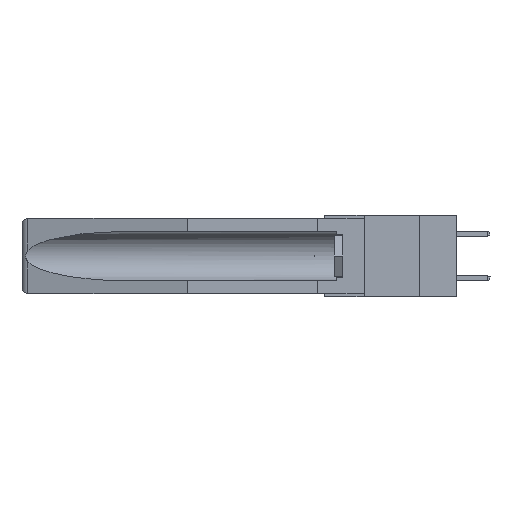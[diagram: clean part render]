
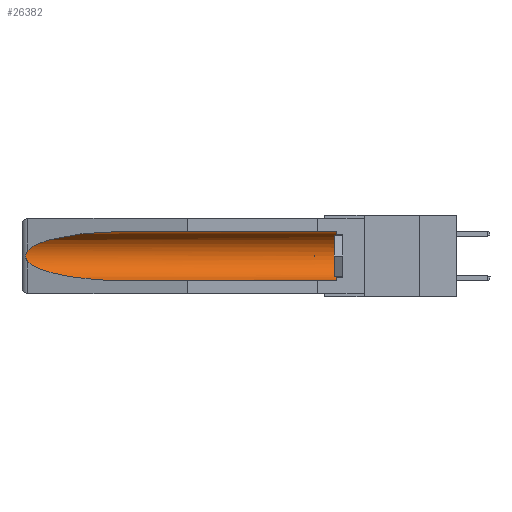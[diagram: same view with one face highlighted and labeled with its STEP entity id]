
A CAD part, left-side view. The second image highlights one B-rep face of the part: STEP entity #26382.
In plain terms, the highlighted cylindrical face has radius 2.857 mm (diameter 5.715 mm), a partial arc.
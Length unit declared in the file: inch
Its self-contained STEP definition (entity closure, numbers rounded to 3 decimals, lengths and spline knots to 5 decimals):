
#333 = DIRECTION ( 'NONE',  ( 0., 0., 1. ) ) ;
#480 = CARTESIAN_POINT ( 'NONE',  ( 0.155, 1.07973, -0.284 ) ) ;
#573 = EDGE_CURVE ( 'NONE', #24997, #14229, #4166, .T. ) ;
#666 = CARTESIAN_POINT ( 'NONE',  ( 0.26537, 1.52718, -0.14972 ) ) ;
#748 = VECTOR ( 'NONE', #4644, 39.37008 ) ;
#827 = LINE ( 'NONE', #33264, #28875 ) ;
#837 = ORIENTED_EDGE ( 'NONE', *, *, #14460, .T. ) ;
#1268 = CARTESIAN_POINT ( 'NONE',  ( 0.26537, 1.52718, -0.19328 ) ) ;
#1581 = CARTESIAN_POINT ( 'NONE',  ( 0.155, 0.126, -0.059 ) ) ;
#2480 = CARTESIAN_POINT ( 'NONE',  ( 0.21114, 1.30732, -0.059 ) ) ;
#2602 = CARTESIAN_POINT ( 'NONE',  ( 0.26537, 1.52718, -0.14972 ) ) ;
#2837 = DIRECTION ( 'NONE',  ( 0., 1., 0. ) ) ;
#2923 = VERTEX_POINT ( 'NONE', #25263 ) ;
#3220 = CARTESIAN_POINT ( 'NONE',  ( 0.21114, 1.30732, -0.284 ) ) ;
#3345 = EDGE_LOOP ( 'NONE', ( #3747, #5036, #6956, #11743, #837, #9358 ) ) ;
#3747 = ORIENTED_EDGE ( 'NONE', *, *, #24088, .T. ) ;
#3888 = CARTESIAN_POINT ( 'NONE',  ( 0.2673, 1.53269, -0.17917 ) ) ;
#4044 = AXIS2_PLACEMENT_3D ( 'NONE', #8190, #2837, #333 ) ;
#4166 = LINE ( 'NONE', #21250, #748 ) ;
#4644 = DIRECTION ( 'NONE',  ( 0., 1., 0. ) ) ;
#5036 = ORIENTED_EDGE ( 'NONE', *, *, #24424, .T. ) ;
#5671 =( BOUNDED_CURVE ( )  B_SPLINE_CURVE ( 3, ( #16665, #25270, #3220, #480 ),
 .UNSPECIFIED., .F., .F. ) 
 B_SPLINE_CURVE_WITH_KNOTS ( ( 4, 4 ),
 ( 0.1948, 1.5708 ),
 .UNSPECIFIED. ) 
 CURVE ( )  GEOMETRIC_REPRESENTATION_ITEM ( )  RATIONAL_B_SPLINE_CURVE ( ( 1., 0.848, 0.848, 1. ) ) 
 REPRESENTATION_ITEM ( '' )  );
#6105 =( BOUNDED_CURVE ( )  B_SPLINE_CURVE ( 3, ( #16149, #2480, #35121, #2602 ),
 .UNSPECIFIED., .F., .F. ) 
 B_SPLINE_CURVE_WITH_KNOTS ( ( 4, 4 ),
 ( 4.71239, 6.08839 ),
 .UNSPECIFIED. ) 
 CURVE ( )  GEOMETRIC_REPRESENTATION_ITEM ( )  RATIONAL_B_SPLINE_CURVE ( ( 1., 0.848, 0.848, 1. ) ) 
 REPRESENTATION_ITEM ( '' )  );
#6149 = CARTESIAN_POINT ( 'NONE',  ( 0.2673, 1.5327, -0.16383 ) ) ;
#6956 = ORIENTED_EDGE ( 'NONE', *, *, #23703, .T. ) ;
#8190 = CARTESIAN_POINT ( 'NONE',  ( 0.155, -0.30754, -0.1715 ) ) ;
#9358 = ORIENTED_EDGE ( 'NONE', *, *, #29932, .T. ) ;
#10224 = FACE_OUTER_BOUND ( 'NONE', #3345, .T. ) ;
#10238 = DIRECTION ( 'NONE',  ( 0., 0., 1. ) ) ;
#11611 = CARTESIAN_POINT ( 'NONE',  ( 0.26597, 1.52961, -0.15275 ) ) ;
#11743 = ORIENTED_EDGE ( 'NONE', *, *, #573, .F. ) ;
#12183 = CARTESIAN_POINT ( 'NONE',  ( 0.2675, 1.53308, -0.16763 ) ) ;
#13424 = AXIS2_PLACEMENT_3D ( 'NONE', #15716, #26491, #10238 ) ;
#13740 = VERTEX_POINT ( 'NONE', #20653 ) ;
#14229 = VERTEX_POINT ( 'NONE', #17162 ) ;
#14460 = EDGE_CURVE ( 'NONE', #24997, #35074, #27917, .T. ) ;
#15716 = CARTESIAN_POINT ( 'NONE',  ( 0.155, 0.126, -0.1715 ) ) ;
#16149 = CARTESIAN_POINT ( 'NONE',  ( 0.155, 1.07973, -0.059 ) ) ;
#16595 = CYLINDRICAL_SURFACE ( 'NONE', #4044, 0.1125 ) ;
#16665 = CARTESIAN_POINT ( 'NONE',  ( 0.26537, 1.52718, -0.19328 ) ) ;
#17162 = CARTESIAN_POINT ( 'NONE',  ( 0.155, 1.07973, -0.284 ) ) ;
#17268 = DIRECTION ( 'NONE',  ( 0., 1., 0. ) ) ;
#18860 = VERTEX_POINT ( 'NONE', #27273 ) ;
#20569 = CARTESIAN_POINT ( 'NONE',  ( 0.155, 0.126, -0.284 ) ) ;
#20653 = CARTESIAN_POINT ( 'NONE',  ( 0.155, 1.07973, -0.059 ) ) ;
#21250 = CARTESIAN_POINT ( 'NONE',  ( 0.155, -0.30754, -0.284 ) ) ;
#22376 = CARTESIAN_POINT ( 'NONE',  ( 0.26654, 1.53092, -0.15636 ) ) ;
#23703 = EDGE_CURVE ( 'NONE', #18860, #14229, #5671, .T. ) ;
#24088 = EDGE_CURVE ( 'NONE', #13740, #2923, #6105, .T. ) ;
#24424 = EDGE_CURVE ( 'NONE', #2923, #18860, #34598, .T. ) ;
#24997 = VERTEX_POINT ( 'NONE', #20569 ) ;
#25263 = CARTESIAN_POINT ( 'NONE',  ( 0.26537, 1.52718, -0.14972 ) ) ;
#25270 = CARTESIAN_POINT ( 'NONE',  ( 0.25451, 1.48313, -0.24835 ) ) ;
#26382 = ADVANCED_FACE ( 'NONE', ( #10224 ), #16595, .F. ) ;
#26491 = DIRECTION ( 'NONE',  ( 0., -1., 0. ) ) ;
#27273 = CARTESIAN_POINT ( 'NONE',  ( 0.26537, 1.52718, -0.19328 ) ) ;
#27917 = CIRCLE ( 'NONE', #13424, 0.1125 ) ;
#28449 = CARTESIAN_POINT ( 'NONE',  ( 0.26597, 1.5296, -0.19026 ) ) ;
#28875 = VECTOR ( 'NONE', #17268, 39.37008 ) ;
#29932 = EDGE_CURVE ( 'NONE', #35074, #13740, #827, .T. ) ;
#31425 = CARTESIAN_POINT ( 'NONE',  ( 0.2675, 1.53308, -0.17534 ) ) ;
#33264 = CARTESIAN_POINT ( 'NONE',  ( 0.155, -0.30754, -0.059 ) ) ;
#34150 = CARTESIAN_POINT ( 'NONE',  ( 0.26655, 1.53094, -0.18657 ) ) ;
#34598 = B_SPLINE_CURVE_WITH_KNOTS ( 'NONE', 3,
 ( #666, #11611, #22376, #6149, #12183, #31425, #3888, #34150, #28449, #1268 ),
 .UNSPECIFIED., .F., .F.,
 ( 4, 2, 2, 2, 4 ),
 ( 0., 0.00029, 0.00058, 0.00087, 0.00117 ),
 .UNSPECIFIED. ) ;
#35074 = VERTEX_POINT ( 'NONE', #1581 ) ;
#35121 = CARTESIAN_POINT ( 'NONE',  ( 0.25451, 1.48313, -0.09465 ) ) ;
